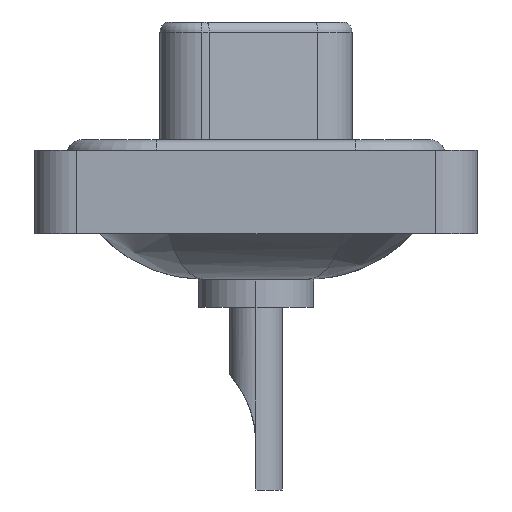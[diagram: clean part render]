
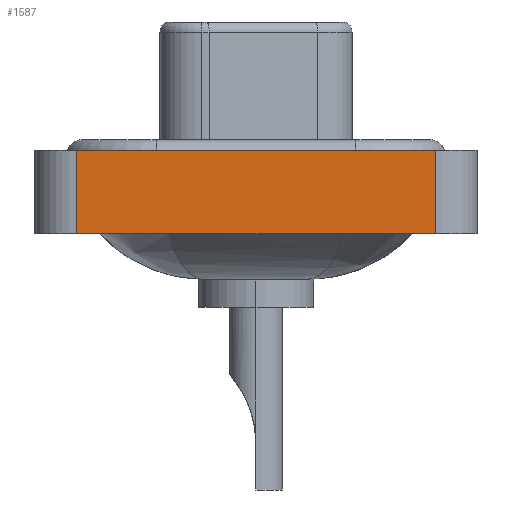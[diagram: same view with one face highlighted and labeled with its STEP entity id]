
A CAD part, left-side view. The second image highlights one B-rep face of the part: STEP entity #1587.
In plain terms, the highlighted planar face has unit normal (-1, 0, 0).
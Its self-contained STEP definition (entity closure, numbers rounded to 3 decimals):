
#158 = DIRECTION ( 'NONE',  ( 0., -1., 0. ) ) ;
#269 = ORIENTED_EDGE ( 'NONE', *, *, #5085, .F. ) ;
#296 = CARTESIAN_POINT ( 'NONE',  ( -7.3, -8.55, -3.6 ) ) ;
#478 = EDGE_LOOP ( 'NONE', ( #3623, #15204, #269, #14375 ) ) ;
#1411 = VERTEX_POINT ( 'NONE', #16020 ) ;
#1587 = ADVANCED_FACE ( 'NONE', ( #6600 ), #2889, .T. ) ;
#1690 = VERTEX_POINT ( 'NONE', #14834 ) ;
#1999 = VERTEX_POINT ( 'NONE', #11013 ) ;
#2889 = PLANE ( 'NONE',  #10669 ) ;
#3051 = VECTOR ( 'NONE', #158, 1000. ) ;
#3528 = LINE ( 'NONE', #13793, #15753 ) ;
#3623 = ORIENTED_EDGE ( 'NONE', *, *, #9813, .T. ) ;
#4170 = VECTOR ( 'NONE', #16439, 1000. ) ;
#4318 = DIRECTION ( 'NONE',  ( 0., 0., 1. ) ) ;
#5085 = EDGE_CURVE ( 'NONE', #1411, #1690, #14073, .T. ) ;
#5527 = EDGE_CURVE ( 'NONE', #1690, #1999, #3528, .T. ) ;
#6299 = CARTESIAN_POINT ( 'NONE',  ( -7.3, -8.55, -3.6 ) ) ;
#6600 = FACE_OUTER_BOUND ( 'NONE', #478, .T. ) ;
#7655 = VERTEX_POINT ( 'NONE', #6299 ) ;
#7703 = LINE ( 'NONE', #296, #10668 ) ;
#7814 = LINE ( 'NONE', #11745, #3051 ) ;
#9813 = EDGE_CURVE ( 'NONE', #7655, #1999, #7703, .T. ) ;
#10668 = VECTOR ( 'NONE', #11555, 1000. ) ;
#10669 = AXIS2_PLACEMENT_3D ( 'NONE', #12986, #15844, #4318 ) ;
#11013 = CARTESIAN_POINT ( 'NONE',  ( -7.3, -8.55, 0.4 ) ) ;
#11555 = DIRECTION ( 'NONE',  ( 0., 0., 1. ) ) ;
#11745 = CARTESIAN_POINT ( 'NONE',  ( -7.3, -8.55, -3.6 ) ) ;
#12452 = CARTESIAN_POINT ( 'NONE',  ( -7.3, 8.55, -3.6 ) ) ;
#12518 = DIRECTION ( 'NONE',  ( 0., -1., 0. ) ) ;
#12986 = CARTESIAN_POINT ( 'NONE',  ( -7.3, -8.55, -3.6 ) ) ;
#13793 = CARTESIAN_POINT ( 'NONE',  ( -7.3, -8.55, 0.4 ) ) ;
#14073 = LINE ( 'NONE', #12452, #4170 ) ;
#14375 = ORIENTED_EDGE ( 'NONE', *, *, #15371, .T. ) ;
#14834 = CARTESIAN_POINT ( 'NONE',  ( -7.3, 8.55, 0.4 ) ) ;
#15204 = ORIENTED_EDGE ( 'NONE', *, *, #5527, .F. ) ;
#15371 = EDGE_CURVE ( 'NONE', #1411, #7655, #7814, .T. ) ;
#15753 = VECTOR ( 'NONE', #12518, 1000. ) ;
#15844 = DIRECTION ( 'NONE',  ( -1., 0., 0. ) ) ;
#16020 = CARTESIAN_POINT ( 'NONE',  ( -7.3, 8.55, -3.6 ) ) ;
#16439 = DIRECTION ( 'NONE',  ( 0., 0., 1. ) ) ;
